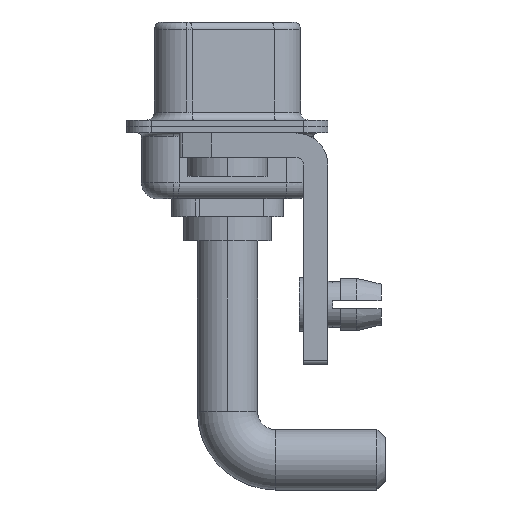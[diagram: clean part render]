
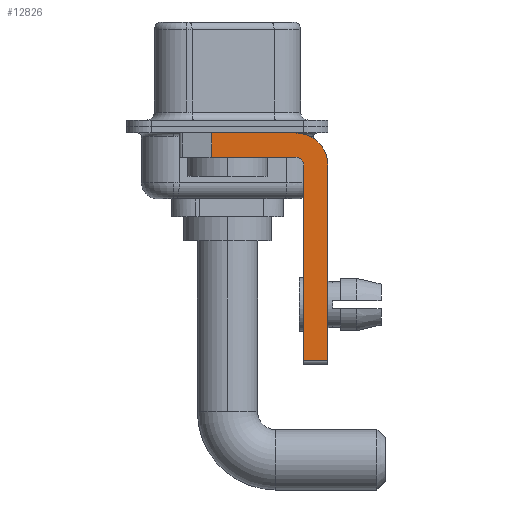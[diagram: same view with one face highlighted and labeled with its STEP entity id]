
A CAD part, left-side view. The second image highlights one B-rep face of the part: STEP entity #12826.
In plain terms, the highlighted planar face has unit normal (-1, 0, 0).
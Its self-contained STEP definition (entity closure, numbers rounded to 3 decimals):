
#54 = CARTESIAN_POINT ( 'NONE',  ( -2.9, -6.25, -2.4 ) ) ;
#342 = VERTEX_POINT ( 'NONE', #11301 ) ;
#510 = CARTESIAN_POINT ( 'NONE',  ( -2.9, 0.978, -1.9 ) ) ;
#635 = DIRECTION ( 'NONE',  ( 1., 0., 0. ) ) ;
#1206 = LINE ( 'NONE', #13947, #13807 ) ;
#1629 = VERTEX_POINT ( 'NONE', #13330 ) ;
#2313 = EDGE_CURVE ( 'NONE', #1629, #7938, #4827, .T. ) ;
#2410 = AXIS2_PLACEMENT_3D ( 'NONE', #3832, #15471, #2422 ) ;
#2422 = DIRECTION ( 'NONE',  ( 0., 0., -1. ) ) ;
#2692 = ORIENTED_EDGE ( 'NONE', *, *, #14314, .F. ) ;
#2796 = EDGE_CURVE ( 'NONE', #342, #12703, #7204, .T. ) ;
#2819 = EDGE_CURVE ( 'NONE', #10717, #5383, #11539, .T. ) ;
#2858 = DIRECTION ( 'NONE',  ( 0., 0., -1. ) ) ;
#3622 = CIRCLE ( 'NONE', #2410, 2. ) ;
#3832 = CARTESIAN_POINT ( 'NONE',  ( -2.9, -4.25, -2.4 ) ) ;
#3877 = VECTOR ( 'NONE', #2858, 1000. ) ;
#3942 = DIRECTION ( 'NONE',  ( 0., 1., 0. ) ) ;
#4193 = VECTOR ( 'NONE', #10817, 1000. ) ;
#4372 = DIRECTION ( 'NONE',  ( 0., -1., 0. ) ) ;
#4447 = ORIENTED_EDGE ( 'NONE', *, *, #2819, .F. ) ;
#4476 = CARTESIAN_POINT ( 'NONE',  ( -2.9, 0.978, -0.4 ) ) ;
#4666 = CARTESIAN_POINT ( 'NONE',  ( -2.9, -4.75, -14.55 ) ) ;
#4827 = CIRCLE ( 'NONE', #9629, 0.5 ) ;
#5383 = VERTEX_POINT ( 'NONE', #9004 ) ;
#6514 = VECTOR ( 'NONE', #14397, 1000. ) ;
#6760 = ORIENTED_EDGE ( 'NONE', *, *, #2796, .F. ) ;
#7204 = LINE ( 'NONE', #54, #3877 ) ;
#7938 = VERTEX_POINT ( 'NONE', #13217 ) ;
#8536 = EDGE_CURVE ( 'NONE', #10717, #10917, #12879, .T. ) ;
#8627 = CARTESIAN_POINT ( 'NONE',  ( -2.9, 0.978, -1.9 ) ) ;
#8913 = DIRECTION ( 'NONE',  ( 0., 0., 1. ) ) ;
#9004 = CARTESIAN_POINT ( 'NONE',  ( -2.9, -4.25, -0.4 ) ) ;
#9298 = CARTESIAN_POINT ( 'NONE',  ( -2.9, -4.25, -2.4 ) ) ;
#9629 = AXIS2_PLACEMENT_3D ( 'NONE', #17348, #16135, #8913 ) ;
#10049 = LINE ( 'NONE', #12880, #10308 ) ;
#10296 = ORIENTED_EDGE ( 'NONE', *, *, #12529, .F. ) ;
#10308 = VECTOR ( 'NONE', #11461, 1000. ) ;
#10434 = EDGE_LOOP ( 'NONE', ( #4447, #15248, #10296, #17938, #14901, #12710, #6760, #2692 ) ) ;
#10717 = VERTEX_POINT ( 'NONE', #4476 ) ;
#10817 = DIRECTION ( 'NONE',  ( 0., -1., 0. ) ) ;
#10838 = VERTEX_POINT ( 'NONE', #4666 ) ;
#10917 = VERTEX_POINT ( 'NONE', #510 ) ;
#11301 = CARTESIAN_POINT ( 'NONE',  ( -2.9, -6.25, -2.4 ) ) ;
#11461 = DIRECTION ( 'NONE',  ( 0., 0., 1. ) ) ;
#11539 = LINE ( 'NONE', #17325, #12663 ) ;
#12001 = AXIS2_PLACEMENT_3D ( 'NONE', #9298, #635, #16156 ) ;
#12529 = EDGE_CURVE ( 'NONE', #7938, #10917, #1206, .T. ) ;
#12663 = VECTOR ( 'NONE', #4372, 1000. ) ;
#12703 = VERTEX_POINT ( 'NONE', #14341 ) ;
#12710 = ORIENTED_EDGE ( 'NONE', *, *, #12982, .T. ) ;
#12826 = ADVANCED_FACE ( 'NONE', ( #18009 ), #13564, .F. ) ;
#12879 = LINE ( 'NONE', #8627, #6514 ) ;
#12880 = CARTESIAN_POINT ( 'NONE',  ( -2.9, -4.75, -14.8 ) ) ;
#12982 = EDGE_CURVE ( 'NONE', #10838, #12703, #18286, .T. ) ;
#13217 = CARTESIAN_POINT ( 'NONE',  ( -2.9, -4.25, -1.9 ) ) ;
#13330 = CARTESIAN_POINT ( 'NONE',  ( -2.9, -4.75, -2.4 ) ) ;
#13564 = PLANE ( 'NONE',  #12001 ) ;
#13807 = VECTOR ( 'NONE', #3942, 1000. ) ;
#13947 = CARTESIAN_POINT ( 'NONE',  ( -2.9, -4.25, -1.9 ) ) ;
#14314 = EDGE_CURVE ( 'NONE', #5383, #342, #3622, .T. ) ;
#14341 = CARTESIAN_POINT ( 'NONE',  ( -2.9, -6.25, -14.55 ) ) ;
#14397 = DIRECTION ( 'NONE',  ( 0., 0., -1. ) ) ;
#14901 = ORIENTED_EDGE ( 'NONE', *, *, #16493, .F. ) ;
#15248 = ORIENTED_EDGE ( 'NONE', *, *, #8536, .T. ) ;
#15471 = DIRECTION ( 'NONE',  ( 1., 0., 0. ) ) ;
#16135 = DIRECTION ( 'NONE',  ( -1., 0., 0. ) ) ;
#16156 = DIRECTION ( 'NONE',  ( 0., 0., -1. ) ) ;
#16493 = EDGE_CURVE ( 'NONE', #10838, #1629, #10049, .T. ) ;
#17325 = CARTESIAN_POINT ( 'NONE',  ( -2.9, 3., -0.4 ) ) ;
#17348 = CARTESIAN_POINT ( 'NONE',  ( -2.9, -4.25, -2.4 ) ) ;
#17938 = ORIENTED_EDGE ( 'NONE', *, *, #2313, .F. ) ;
#18009 = FACE_OUTER_BOUND ( 'NONE', #10434, .T. ) ;
#18286 = LINE ( 'NONE', #18482, #4193 ) ;
#18482 = CARTESIAN_POINT ( 'NONE',  ( -2.9, -4.25, -14.55 ) ) ;
